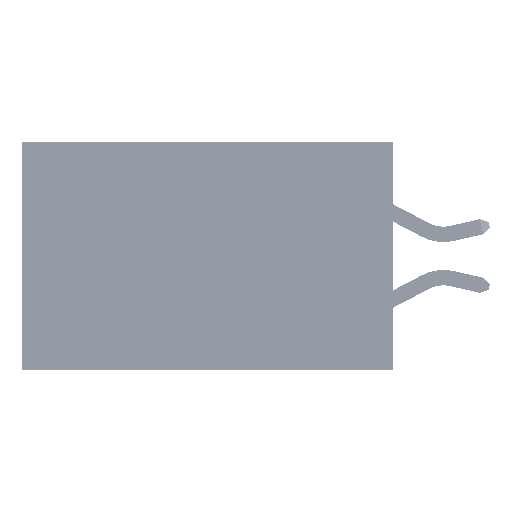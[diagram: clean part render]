
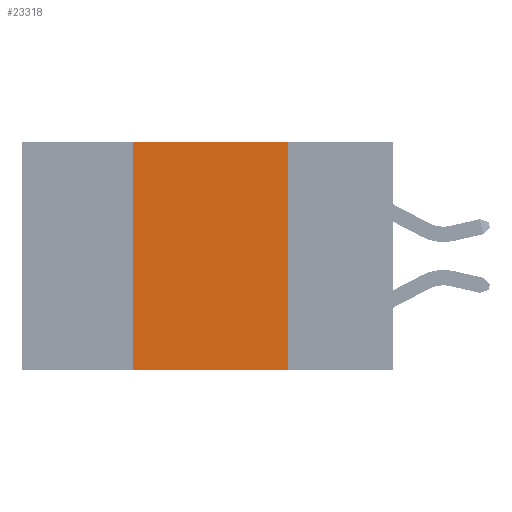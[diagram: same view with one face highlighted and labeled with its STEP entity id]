
A CAD part, left-side view. The second image highlights one B-rep face of the part: STEP entity #23318.
In plain terms, the highlighted planar face has unit normal (-1, 0, 0).
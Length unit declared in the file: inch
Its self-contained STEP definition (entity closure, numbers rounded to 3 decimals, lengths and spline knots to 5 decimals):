
#593 = DIRECTION ( 'NONE',  ( 1., 0., 0. ) ) ;
#775 = ORIENTED_EDGE ( 'NONE', *, *, #46480, .F. ) ;
#1188 = VERTEX_POINT ( 'NONE', #18589 ) ;
#3118 = DIRECTION ( 'NONE',  ( 0., -1., 0. ) ) ;
#3763 = CARTESIAN_POINT ( 'NONE',  ( 0., 0.17, 0. ) ) ;
#8119 = DIRECTION ( 'NONE',  ( 0., 0., -1. ) ) ;
#9082 = LINE ( 'NONE', #34885, #39588 ) ;
#9957 = VERTEX_POINT ( 'NONE', #10921 ) ;
#10921 = CARTESIAN_POINT ( 'NONE',  ( 0., 0.42, -0.37 ) ) ;
#11528 = FACE_OUTER_BOUND ( 'NONE', #25039, .T. ) ;
#11567 = LINE ( 'NONE', #22222, #29527 ) ;
#13861 = LINE ( 'NONE', #3763, #16768 ) ;
#15500 = DIRECTION ( 'NONE',  ( 0., 0., -1. ) ) ;
#15630 = EDGE_CURVE ( 'NONE', #9957, #36436, #45260, .T. ) ;
#16768 = VECTOR ( 'NONE', #15500, 39.37008 ) ;
#18184 = CARTESIAN_POINT ( 'NONE',  ( 0., 0.42, 0. ) ) ;
#18589 = CARTESIAN_POINT ( 'NONE',  ( 0., 0.17, -0.37 ) ) ;
#22100 = CARTESIAN_POINT ( 'NONE',  ( 0., 0.17, 0. ) ) ;
#22222 = CARTESIAN_POINT ( 'NONE',  ( 0., 0.6, -0.37 ) ) ;
#23047 = EDGE_CURVE ( 'NONE', #9957, #1188, #11567, .T. ) ;
#23318 = ADVANCED_FACE ( 'NONE', ( #11528 ), #46370, .F. ) ;
#25039 = EDGE_LOOP ( 'NONE', ( #48647, #775, #33968, #33811 ) ) ;
#29527 = VECTOR ( 'NONE', #3118, 39.37008 ) ;
#31193 = DIRECTION ( 'NONE',  ( 0., -1., 0. ) ) ;
#32353 = CARTESIAN_POINT ( 'NONE',  ( 0., 0.42, 0. ) ) ;
#33811 = ORIENTED_EDGE ( 'NONE', *, *, #23047, .T. ) ;
#33968 = ORIENTED_EDGE ( 'NONE', *, *, #15630, .F. ) ;
#34885 = CARTESIAN_POINT ( 'NONE',  ( 0., 0.6, 0. ) ) ;
#35136 = VECTOR ( 'NONE', #35879, 39.37008 ) ;
#35879 = DIRECTION ( 'NONE',  ( 0., 0., 1. ) ) ;
#36436 = VERTEX_POINT ( 'NONE', #18184 ) ;
#39588 = VECTOR ( 'NONE', #31193, 39.37008 ) ;
#40138 = AXIS2_PLACEMENT_3D ( 'NONE', #46689, #593, #8119 ) ;
#43396 = EDGE_CURVE ( 'NONE', #44500, #1188, #13861, .T. ) ;
#44500 = VERTEX_POINT ( 'NONE', #22100 ) ;
#45260 = LINE ( 'NONE', #32353, #35136 ) ;
#46370 = PLANE ( 'NONE',  #40138 ) ;
#46480 = EDGE_CURVE ( 'NONE', #36436, #44500, #9082, .T. ) ;
#46689 = CARTESIAN_POINT ( 'NONE',  ( 0., 0.6, 0. ) ) ;
#48647 = ORIENTED_EDGE ( 'NONE', *, *, #43396, .F. ) ;
